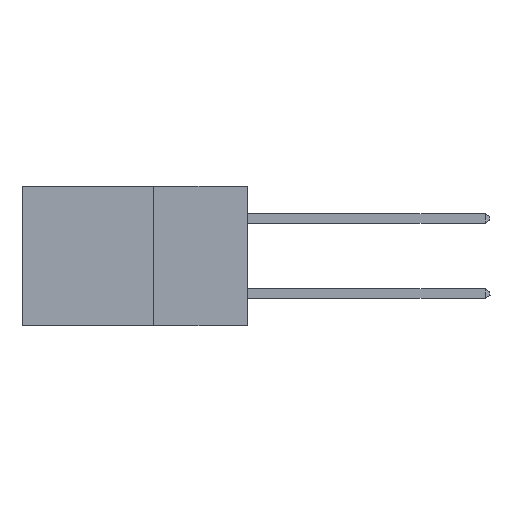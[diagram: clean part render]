
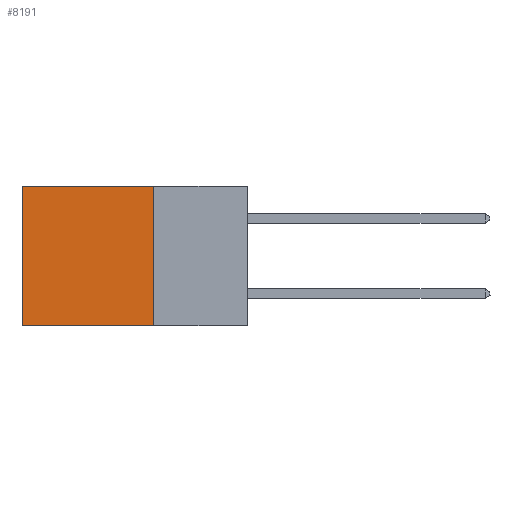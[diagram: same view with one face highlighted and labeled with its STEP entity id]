
A CAD part, left-side view. The second image highlights one B-rep face of the part: STEP entity #8191.
In plain terms, the highlighted planar face has unit normal (-1, 0, 0).
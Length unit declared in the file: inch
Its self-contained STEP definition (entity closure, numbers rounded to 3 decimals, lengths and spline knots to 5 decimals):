
#10 = LINE ( 'NONE', #4612, #11964 ) ;
#915 = CARTESIAN_POINT ( 'NONE',  ( 0.298, 0.25, 0. ) ) ;
#1569 = LINE ( 'NONE', #17963, #18647 ) ;
#2054 = FACE_OUTER_BOUND ( 'NONE', #10515, .T. ) ;
#2300 = DIRECTION ( 'NONE',  ( 0., 0., -1. ) ) ;
#3005 = LINE ( 'NONE', #915, #10357 ) ;
#3681 = ORIENTED_EDGE ( 'NONE', *, *, #16187, .T. ) ;
#4069 = AXIS2_PLACEMENT_3D ( 'NONE', #15378, #11086, #2300 ) ;
#4127 = ORIENTED_EDGE ( 'NONE', *, *, #8461, .T. ) ;
#4612 = CARTESIAN_POINT ( 'NONE',  ( 0.298, 0.25, 0. ) ) ;
#4817 = DIRECTION ( 'NONE',  ( 0., 1., 0. ) ) ;
#4925 = CARTESIAN_POINT ( 'NONE',  ( 0.298, 0.6, -0.37 ) ) ;
#6426 = CARTESIAN_POINT ( 'NONE',  ( 0.298, 0.25, -0.37 ) ) ;
#8118 = ORIENTED_EDGE ( 'NONE', *, *, #18298, .F. ) ;
#8191 = ADVANCED_FACE ( 'NONE', ( #2054 ), #11022, .F. ) ;
#8375 = DIRECTION ( 'NONE',  ( 0., 0., -1. ) ) ;
#8461 = EDGE_CURVE ( 'NONE', #14400, #15225, #1569, .T. ) ;
#8665 = VECTOR ( 'NONE', #4817, 39.37008 ) ;
#9024 = DIRECTION ( 'NONE',  ( 0., 1., 0. ) ) ;
#9137 = CARTESIAN_POINT ( 'NONE',  ( 0.298, 0.25, 0. ) ) ;
#9467 = CARTESIAN_POINT ( 'NONE',  ( 0.298, 0.25, -0.37 ) ) ;
#10071 = VERTEX_POINT ( 'NONE', #9467 ) ;
#10357 = VECTOR ( 'NONE', #8375, 39.37008 ) ;
#10515 = EDGE_LOOP ( 'NONE', ( #4127, #8118, #10794, #3681 ) ) ;
#10794 = ORIENTED_EDGE ( 'NONE', *, *, #16571, .F. ) ;
#11022 = PLANE ( 'NONE',  #4069 ) ;
#11086 = DIRECTION ( 'NONE',  ( 1., 0., 0. ) ) ;
#11964 = VECTOR ( 'NONE', #9024, 39.37008 ) ;
#12233 = DIRECTION ( 'NONE',  ( 0., 0., -1. ) ) ;
#12249 = VERTEX_POINT ( 'NONE', #9137 ) ;
#12565 = LINE ( 'NONE', #6426, #8665 ) ;
#14400 = VERTEX_POINT ( 'NONE', #15345 ) ;
#15225 = VERTEX_POINT ( 'NONE', #4925 ) ;
#15345 = CARTESIAN_POINT ( 'NONE',  ( 0.298, 0.6, 0. ) ) ;
#15378 = CARTESIAN_POINT ( 'NONE',  ( 0.298, 0.25, 0. ) ) ;
#16187 = EDGE_CURVE ( 'NONE', #12249, #14400, #10, .T. ) ;
#16571 = EDGE_CURVE ( 'NONE', #12249, #10071, #3005, .T. ) ;
#17963 = CARTESIAN_POINT ( 'NONE',  ( 0.298, 0.6, 0. ) ) ;
#18298 = EDGE_CURVE ( 'NONE', #10071, #15225, #12565, .T. ) ;
#18647 = VECTOR ( 'NONE', #12233, 39.37008 ) ;
